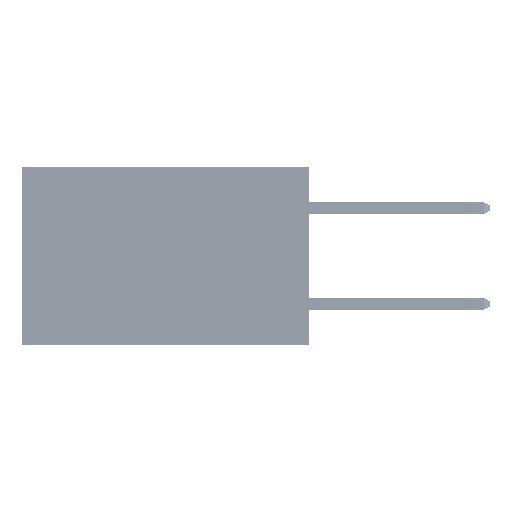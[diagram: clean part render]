
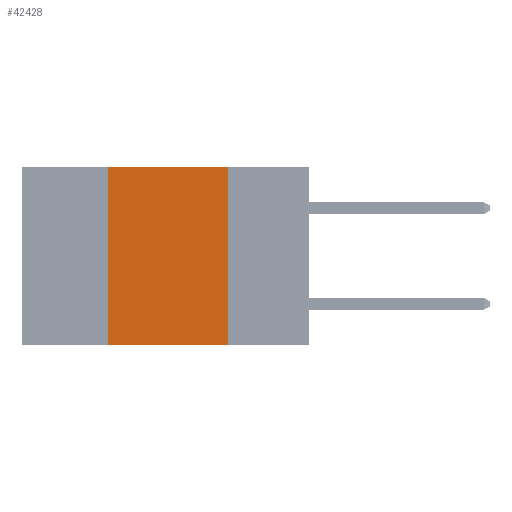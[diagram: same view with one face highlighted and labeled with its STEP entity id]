
A CAD part, left-side view. The second image highlights one B-rep face of the part: STEP entity #42428.
In plain terms, the highlighted planar face has unit normal (-1, 0, 0).
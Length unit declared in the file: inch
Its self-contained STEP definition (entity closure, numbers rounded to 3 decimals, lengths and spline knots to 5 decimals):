
#1658 = EDGE_CURVE ( 'NONE', #8281, #11526, #24829, .T. ) ;
#1899 = AXIS2_PLACEMENT_3D ( 'NONE', #3495, #11794, #43192 ) ;
#3495 = CARTESIAN_POINT ( 'NONE',  ( 0., 0.6, 0. ) ) ;
#4351 = CARTESIAN_POINT ( 'NONE',  ( 0., 0.17, 0. ) ) ;
#6760 = CARTESIAN_POINT ( 'NONE',  ( 0., 0.6, -0.37 ) ) ;
#7138 = CARTESIAN_POINT ( 'NONE',  ( 0., 0.42, -0.37 ) ) ;
#8281 = VERTEX_POINT ( 'NONE', #4351 ) ;
#9710 = LINE ( 'NONE', #41087, #44864 ) ;
#10022 = CARTESIAN_POINT ( 'NONE',  ( 0., 0.17, 0. ) ) ;
#11526 = VERTEX_POINT ( 'NONE', #17190 ) ;
#11794 = DIRECTION ( 'NONE',  ( 1., 0., 0. ) ) ;
#11989 = CARTESIAN_POINT ( 'NONE',  ( 0., 0.42, 0. ) ) ;
#13542 = ORIENTED_EDGE ( 'NONE', *, *, #34643, .F. ) ;
#14004 = DIRECTION ( 'NONE',  ( 0., 0., -1. ) ) ;
#17190 = CARTESIAN_POINT ( 'NONE',  ( 0., 0.17, -0.37 ) ) ;
#17321 = DIRECTION ( 'NONE',  ( 0., -1., 0. ) ) ;
#18192 = EDGE_LOOP ( 'NONE', ( #49716, #13542, #30412, #19698 ) ) ;
#19401 = VECTOR ( 'NONE', #40072, 39.37008 ) ;
#19698 = ORIENTED_EDGE ( 'NONE', *, *, #26748, .T. ) ;
#24829 = LINE ( 'NONE', #10022, #39027 ) ;
#26632 = DIRECTION ( 'NONE',  ( 0., -1., 0. ) ) ;
#26748 = EDGE_CURVE ( 'NONE', #41135, #11526, #35016, .T. ) ;
#28033 = FACE_OUTER_BOUND ( 'NONE', #18192, .T. ) ;
#30116 = VECTOR ( 'NONE', #26632, 39.37008 ) ;
#30412 = ORIENTED_EDGE ( 'NONE', *, *, #36408, .F. ) ;
#31083 = VERTEX_POINT ( 'NONE', #50802 ) ;
#34643 = EDGE_CURVE ( 'NONE', #31083, #8281, #9710, .T. ) ;
#35016 = LINE ( 'NONE', #6760, #30116 ) ;
#36408 = EDGE_CURVE ( 'NONE', #41135, #31083, #43449, .T. ) ;
#39027 = VECTOR ( 'NONE', #14004, 39.37008 ) ;
#40072 = DIRECTION ( 'NONE',  ( 0., 0., 1. ) ) ;
#41087 = CARTESIAN_POINT ( 'NONE',  ( 0., 0.6, 0. ) ) ;
#41135 = VERTEX_POINT ( 'NONE', #7138 ) ;
#42428 = ADVANCED_FACE ( 'NONE', ( #28033 ), #42853, .F. ) ;
#42853 = PLANE ( 'NONE',  #1899 ) ;
#43192 = DIRECTION ( 'NONE',  ( 0., 0., -1. ) ) ;
#43449 = LINE ( 'NONE', #11989, #19401 ) ;
#44864 = VECTOR ( 'NONE', #17321, 39.37008 ) ;
#49716 = ORIENTED_EDGE ( 'NONE', *, *, #1658, .F. ) ;
#50802 = CARTESIAN_POINT ( 'NONE',  ( 0., 0.42, 0. ) ) ;
